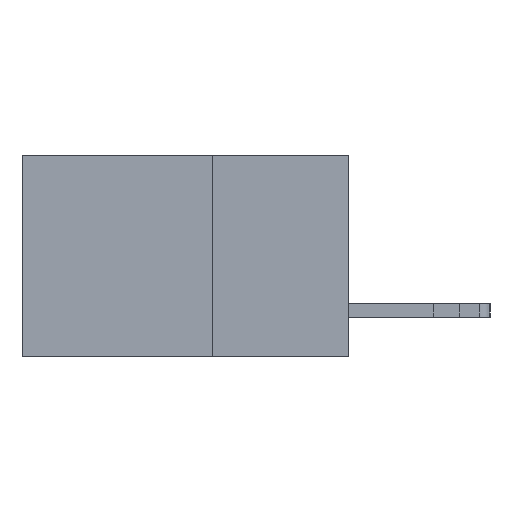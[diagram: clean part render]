
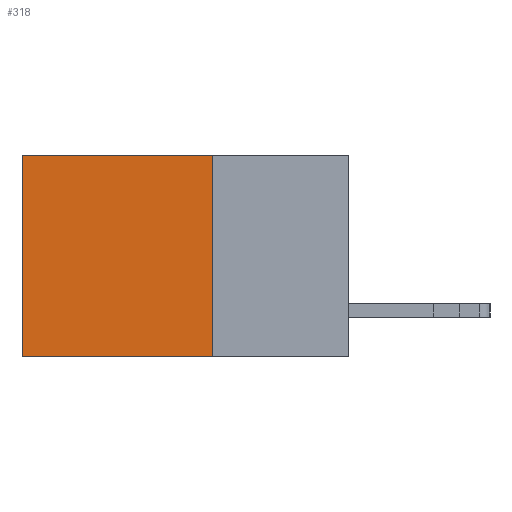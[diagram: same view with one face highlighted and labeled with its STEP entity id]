
A CAD part, left-side view. The second image highlights one B-rep face of the part: STEP entity #318.
In plain terms, the highlighted planar face has unit normal (-1, 0, 0).
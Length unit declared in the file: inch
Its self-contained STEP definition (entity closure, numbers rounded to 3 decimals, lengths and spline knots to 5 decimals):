
#71 = DIRECTION ( 'NONE',  ( 0., 0., -1. ) ) ;
#112 = DIRECTION ( 'NONE',  ( 0., 0., -1. ) ) ;
#258 = VERTEX_POINT ( 'NONE', #641 ) ;
#318 = ADVANCED_FACE ( 'NONE', ( #1563 ), #2965, .F. ) ;
#417 = DIRECTION ( 'NONE',  ( 0., 1., 0. ) ) ;
#641 = CARTESIAN_POINT ( 'NONE',  ( 0.2615, 0.25, 0. ) ) ;
#819 = VECTOR ( 'NONE', #71, 39.37008 ) ;
#1563 = FACE_OUTER_BOUND ( 'NONE', #9341, .T. ) ;
#1682 = CARTESIAN_POINT ( 'NONE',  ( 0.2615, 0.6, -0.37 ) ) ;
#1963 = CARTESIAN_POINT ( 'NONE',  ( 0.2615, 0.6, 0. ) ) ;
#2576 = VECTOR ( 'NONE', #417, 39.37008 ) ;
#2610 = VERTEX_POINT ( 'NONE', #1963 ) ;
#2907 = EDGE_CURVE ( 'NONE', #258, #5220, #6978, .T. ) ;
#2933 = DIRECTION ( 'NONE',  ( 0., 0., -1. ) ) ;
#2965 = PLANE ( 'NONE',  #2994 ) ;
#2976 = CARTESIAN_POINT ( 'NONE',  ( 0.2615, 0.25, -0.37 ) ) ;
#2991 = DIRECTION ( 'NONE',  ( 1., 0., 0. ) ) ;
#2994 = AXIS2_PLACEMENT_3D ( 'NONE', #2976, #2991, #112 ) ;
#3407 = EDGE_CURVE ( 'NONE', #5220, #8779, #4908, .T. ) ;
#4054 = ORIENTED_EDGE ( 'NONE', *, *, #4686, .T. ) ;
#4171 = ORIENTED_EDGE ( 'NONE', *, *, #2907, .F. ) ;
#4202 = ORIENTED_EDGE ( 'NONE', *, *, #3407, .F. ) ;
#4363 = ORIENTED_EDGE ( 'NONE', *, *, #8483, .T. ) ;
#4686 = EDGE_CURVE ( 'NONE', #258, #2610, #7381, .T. ) ;
#4908 = LINE ( 'NONE', #5898, #2576 ) ;
#5220 = VERTEX_POINT ( 'NONE', #8177 ) ;
#5898 = CARTESIAN_POINT ( 'NONE',  ( 0.2615, 0.25, -0.37 ) ) ;
#5929 = CARTESIAN_POINT ( 'NONE',  ( 0.2615, 0.6, -0.37 ) ) ;
#6062 = CARTESIAN_POINT ( 'NONE',  ( 0.2615, 0.25, 0. ) ) ;
#6126 = DIRECTION ( 'NONE',  ( 0., 1., 0. ) ) ;
#6978 = LINE ( 'NONE', #9701, #819 ) ;
#7168 = VECTOR ( 'NONE', #6126, 39.37008 ) ;
#7381 = LINE ( 'NONE', #6062, #7168 ) ;
#7442 = VECTOR ( 'NONE', #2933, 39.37008 ) ;
#8177 = CARTESIAN_POINT ( 'NONE',  ( 0.2615, 0.25, -0.37 ) ) ;
#8483 = EDGE_CURVE ( 'NONE', #2610, #8779, #9231, .T. ) ;
#8779 = VERTEX_POINT ( 'NONE', #1682 ) ;
#9231 = LINE ( 'NONE', #5929, #7442 ) ;
#9341 = EDGE_LOOP ( 'NONE', ( #4363, #4202, #4171, #4054 ) ) ;
#9701 = CARTESIAN_POINT ( 'NONE',  ( 0.2615, 0.25, -0.37 ) ) ;
